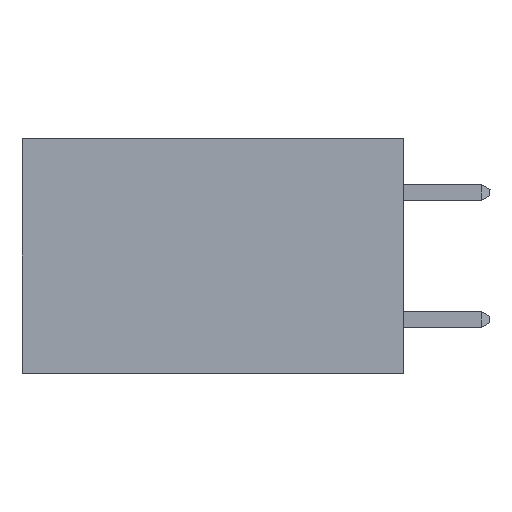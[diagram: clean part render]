
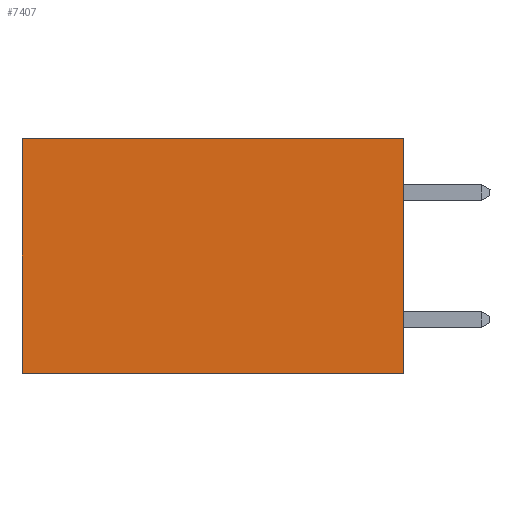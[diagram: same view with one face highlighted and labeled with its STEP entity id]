
A CAD part, left-side view. The second image highlights one B-rep face of the part: STEP entity #7407.
In plain terms, the highlighted planar face has unit normal (-1, 0, 0).
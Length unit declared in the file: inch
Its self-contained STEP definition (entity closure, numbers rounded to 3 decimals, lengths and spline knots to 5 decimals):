
#483 = EDGE_LOOP ( 'NONE', ( #6657, #19669, #9486, #4427 ) ) ;
#542 = CARTESIAN_POINT ( 'NONE',  ( 0.2875, 0., -0.37 ) ) ;
#903 = LINE ( 'NONE', #13642, #5126 ) ;
#1073 = DIRECTION ( 'NONE',  ( 1., 0., 0. ) ) ;
#1116 = VERTEX_POINT ( 'NONE', #542 ) ;
#2038 = DIRECTION ( 'NONE',  ( 0., 0., -1. ) ) ;
#4427 = ORIENTED_EDGE ( 'NONE', *, *, #14759, .T. ) ;
#5005 = CARTESIAN_POINT ( 'NONE',  ( 0.2875, 0.6, 0. ) ) ;
#5126 = VECTOR ( 'NONE', #17588, 39.37008 ) ;
#6657 = ORIENTED_EDGE ( 'NONE', *, *, #18091, .T. ) ;
#6667 = AXIS2_PLACEMENT_3D ( 'NONE', #23868, #1073, #12513 ) ;
#7174 = FACE_OUTER_BOUND ( 'NONE', #483, .T. ) ;
#7226 = EDGE_CURVE ( 'NONE', #1116, #14013, #11978, .T. ) ;
#7407 = ADVANCED_FACE ( 'NONE', ( #7174 ), #18222, .F. ) ;
#8969 = VECTOR ( 'NONE', #19977, 39.37008 ) ;
#9168 = VECTOR ( 'NONE', #12906, 39.37008 ) ;
#9486 = ORIENTED_EDGE ( 'NONE', *, *, #23452, .F. ) ;
#10500 = VECTOR ( 'NONE', #2038, 39.37008 ) ;
#10814 = LINE ( 'NONE', #11797, #10500 ) ;
#11775 = CARTESIAN_POINT ( 'NONE',  ( 0.2875, 0., 0. ) ) ;
#11797 = CARTESIAN_POINT ( 'NONE',  ( 0.2875, 0., 0. ) ) ;
#11854 = LINE ( 'NONE', #5005, #9168 ) ;
#11978 = LINE ( 'NONE', #12374, #8969 ) ;
#12374 = CARTESIAN_POINT ( 'NONE',  ( 0.2875, 0., -0.37 ) ) ;
#12513 = DIRECTION ( 'NONE',  ( 0., 0., -1. ) ) ;
#12906 = DIRECTION ( 'NONE',  ( 0., 0., -1. ) ) ;
#13642 = CARTESIAN_POINT ( 'NONE',  ( 0.2875, 0., 0. ) ) ;
#14013 = VERTEX_POINT ( 'NONE', #19223 ) ;
#14759 = EDGE_CURVE ( 'NONE', #18853, #17621, #903, .T. ) ;
#17588 = DIRECTION ( 'NONE',  ( 0., 1., 0. ) ) ;
#17621 = VERTEX_POINT ( 'NONE', #19316 ) ;
#18091 = EDGE_CURVE ( 'NONE', #17621, #14013, #11854, .T. ) ;
#18222 = PLANE ( 'NONE',  #6667 ) ;
#18853 = VERTEX_POINT ( 'NONE', #11775 ) ;
#19223 = CARTESIAN_POINT ( 'NONE',  ( 0.2875, 0.6, -0.37 ) ) ;
#19316 = CARTESIAN_POINT ( 'NONE',  ( 0.2875, 0.6, 0. ) ) ;
#19669 = ORIENTED_EDGE ( 'NONE', *, *, #7226, .F. ) ;
#19977 = DIRECTION ( 'NONE',  ( 0., 1., 0. ) ) ;
#23452 = EDGE_CURVE ( 'NONE', #18853, #1116, #10814, .T. ) ;
#23868 = CARTESIAN_POINT ( 'NONE',  ( 0.2875, 0., 0. ) ) ;
